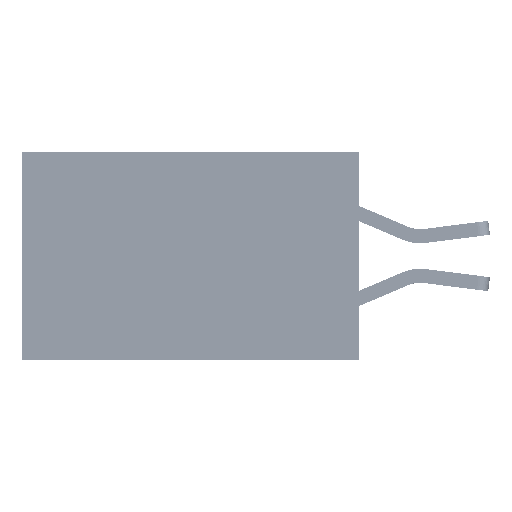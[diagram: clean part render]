
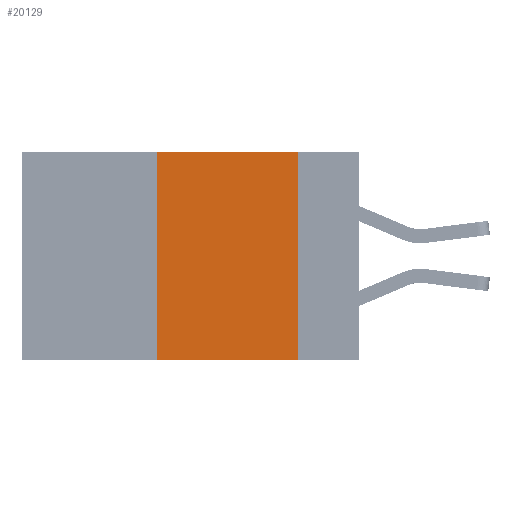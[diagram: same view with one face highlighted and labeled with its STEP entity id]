
A CAD part, left-side view. The second image highlights one B-rep face of the part: STEP entity #20129.
In plain terms, the highlighted planar face has unit normal (-1, 0, 0).
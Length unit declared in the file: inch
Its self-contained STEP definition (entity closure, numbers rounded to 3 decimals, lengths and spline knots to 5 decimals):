
#98 = DIRECTION ( 'NONE',  ( 1., 0., 0. ) ) ;
#258 = CARTESIAN_POINT ( 'NONE',  ( 0., 0.6, 0. ) ) ;
#560 = VERTEX_POINT ( 'NONE', #8622 ) ;
#1736 = EDGE_LOOP ( 'NONE', ( #4533, #46662, #12748, #19946 ) ) ;
#1771 = DIRECTION ( 'NONE',  ( 0., 0., 1. ) ) ;
#2957 = EDGE_CURVE ( 'NONE', #10725, #47026, #13669, .T. ) ;
#4399 = LINE ( 'NONE', #7728, #27730 ) ;
#4533 = ORIENTED_EDGE ( 'NONE', *, *, #49879, .F. ) ;
#5124 = AXIS2_PLACEMENT_3D ( 'NONE', #258, #98, #39338 ) ;
#7522 = PLANE ( 'NONE',  #5124 ) ;
#7728 = CARTESIAN_POINT ( 'NONE',  ( 0., 0.6, -0.37 ) ) ;
#8622 = CARTESIAN_POINT ( 'NONE',  ( 0., 0.36, -0.37 ) ) ;
#10725 = VERTEX_POINT ( 'NONE', #45450 ) ;
#11236 = VECTOR ( 'NONE', #43704, 39.37008 ) ;
#12748 = ORIENTED_EDGE ( 'NONE', *, *, #37455, .F. ) ;
#13424 = CARTESIAN_POINT ( 'NONE',  ( 0., 0.36, 0. ) ) ;
#13669 = LINE ( 'NONE', #43883, #11236 ) ;
#13778 = CARTESIAN_POINT ( 'NONE',  ( 0., 0.11, 0. ) ) ;
#15782 = FACE_OUTER_BOUND ( 'NONE', #1736, .T. ) ;
#15838 = CARTESIAN_POINT ( 'NONE',  ( 0., 0.11, -0.37 ) ) ;
#19946 = ORIENTED_EDGE ( 'NONE', *, *, #50421, .T. ) ;
#20129 = ADVANCED_FACE ( 'NONE', ( #15782 ), #7522, .F. ) ;
#23289 = VECTOR ( 'NONE', #1771, 39.37008 ) ;
#27208 = VERTEX_POINT ( 'NONE', #15838 ) ;
#27365 = CARTESIAN_POINT ( 'NONE',  ( 0., 0.11, 0. ) ) ;
#27683 = DIRECTION ( 'NONE',  ( 0., 0., -1. ) ) ;
#27730 = VECTOR ( 'NONE', #42819, 39.37008 ) ;
#33784 = LINE ( 'NONE', #13424, #23289 ) ;
#37455 = EDGE_CURVE ( 'NONE', #560, #10725, #33784, .T. ) ;
#37673 = LINE ( 'NONE', #27365, #45645 ) ;
#39338 = DIRECTION ( 'NONE',  ( 0., 0., -1. ) ) ;
#42819 = DIRECTION ( 'NONE',  ( 0., -1., 0. ) ) ;
#43704 = DIRECTION ( 'NONE',  ( 0., -1., 0. ) ) ;
#43883 = CARTESIAN_POINT ( 'NONE',  ( 0., 0.6, 0. ) ) ;
#45450 = CARTESIAN_POINT ( 'NONE',  ( 0., 0.36, 0. ) ) ;
#45645 = VECTOR ( 'NONE', #27683, 39.37008 ) ;
#46662 = ORIENTED_EDGE ( 'NONE', *, *, #2957, .F. ) ;
#47026 = VERTEX_POINT ( 'NONE', #13778 ) ;
#49879 = EDGE_CURVE ( 'NONE', #47026, #27208, #37673, .T. ) ;
#50421 = EDGE_CURVE ( 'NONE', #560, #27208, #4399, .T. ) ;
